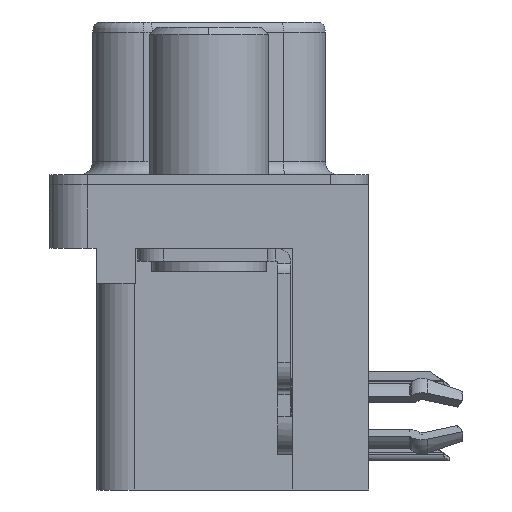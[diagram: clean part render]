
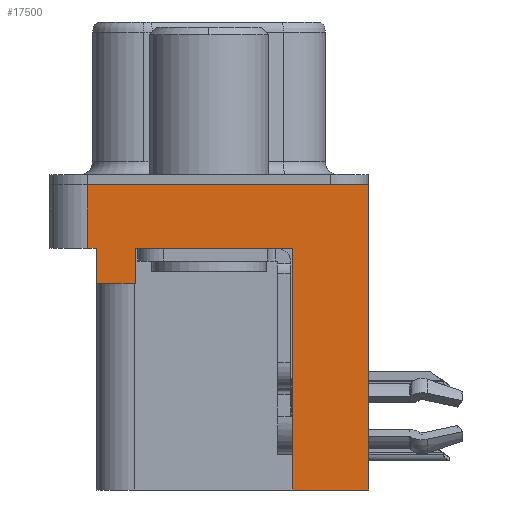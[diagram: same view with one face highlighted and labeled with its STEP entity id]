
A CAD part, left-side view. The second image highlights one B-rep face of the part: STEP entity #17500.
In plain terms, the highlighted planar face has unit normal (-1, 0, 0).
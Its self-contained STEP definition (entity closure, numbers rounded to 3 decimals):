
#219 = AXIS2_PLACEMENT_3D ( 'NONE', #14425, #825, #19557 ) ;
#487 = CARTESIAN_POINT ( 'NONE',  ( -3., 4.775, 0. ) ) ;
#608 = CARTESIAN_POINT ( 'NONE',  ( -3., 4.425, -2.5 ) ) ;
#825 = DIRECTION ( 'NONE',  ( -1., 0., 0. ) ) ;
#910 = VECTOR ( 'NONE', #11393, 1000. ) ;
#1027 = LINE ( 'NONE', #5303, #11777 ) ;
#1289 = ORIENTED_EDGE ( 'NONE', *, *, #22058, .T. ) ;
#1458 = DIRECTION ( 'NONE',  ( 0., -1., 0. ) ) ;
#1572 = EDGE_LOOP ( 'NONE', ( #5381, #14728, #16330, #17282, #4037, #6129, #1289, #3602, #12675, #18749 ) ) ;
#2062 = DIRECTION ( 'NONE',  ( 0., 0., 1. ) ) ;
#2602 = VERTEX_POINT ( 'NONE', #22651 ) ;
#3520 = VERTEX_POINT ( 'NONE', #20927 ) ;
#3602 = ORIENTED_EDGE ( 'NONE', *, *, #14326, .F. ) ;
#4037 = ORIENTED_EDGE ( 'NONE', *, *, #7363, .F. ) ;
#4513 = EDGE_CURVE ( 'NONE', #12724, #22616, #8514, .T. ) ;
#4618 = CARTESIAN_POINT ( 'NONE',  ( -3., -3.295, -12. ) ) ;
#5106 = VECTOR ( 'NONE', #17898, 1000. ) ;
#5303 = CARTESIAN_POINT ( 'NONE',  ( -3., -6.275, -2.5 ) ) ;
#5381 = ORIENTED_EDGE ( 'NONE', *, *, #9587, .F. ) ;
#5887 = CARTESIAN_POINT ( 'NONE',  ( -3., 2.895, -3.9 ) ) ;
#6129 = ORIENTED_EDGE ( 'NONE', *, *, #20632, .T. ) ;
#6624 = DIRECTION ( 'NONE',  ( 0., 1., 0. ) ) ;
#6923 = DIRECTION ( 'NONE',  ( 0., -1., 0. ) ) ;
#6951 = DIRECTION ( 'NONE',  ( 0., 0., 1. ) ) ;
#7041 = CARTESIAN_POINT ( 'NONE',  ( -3., 4.425, -3.9 ) ) ;
#7279 = CARTESIAN_POINT ( 'NONE',  ( -3., -3.295, -12. ) ) ;
#7363 = EDGE_CURVE ( 'NONE', #14541, #21004, #24145, .T. ) ;
#8294 = DIRECTION ( 'NONE',  ( 0., 1., 0. ) ) ;
#8514 = LINE ( 'NONE', #4618, #14204 ) ;
#9392 = EDGE_CURVE ( 'NONE', #18677, #16371, #24678, .T. ) ;
#9587 = EDGE_CURVE ( 'NONE', #16371, #19095, #24375, .T. ) ;
#9686 = CARTESIAN_POINT ( 'NONE',  ( -3., -6.275, 0. ) ) ;
#9701 = FACE_OUTER_BOUND ( 'NONE', #1572, .T. ) ;
#9835 = PLANE ( 'NONE',  #219 ) ;
#9888 = CARTESIAN_POINT ( 'NONE',  ( -3., 4.775, -2.5 ) ) ;
#10728 = VECTOR ( 'NONE', #6923, 1000. ) ;
#11393 = DIRECTION ( 'NONE',  ( 0., 0., 1. ) ) ;
#11777 = VECTOR ( 'NONE', #6951, 1000. ) ;
#11969 = CARTESIAN_POINT ( 'NONE',  ( -3., 4.775, -2.5 ) ) ;
#12283 = CARTESIAN_POINT ( 'NONE',  ( -3., 4.425, -3.9 ) ) ;
#12320 = EDGE_CURVE ( 'NONE', #21004, #18880, #13781, .T. ) ;
#12675 = ORIENTED_EDGE ( 'NONE', *, *, #4513, .F. ) ;
#12724 = VERTEX_POINT ( 'NONE', #24806 ) ;
#12850 = CARTESIAN_POINT ( 'NONE',  ( -3., 2.895, -3.9 ) ) ;
#12912 = CARTESIAN_POINT ( 'NONE',  ( -3., -6.275, 0. ) ) ;
#13331 = EDGE_CURVE ( 'NONE', #18677, #18880, #19086, .T. ) ;
#13781 = LINE ( 'NONE', #22675, #910 ) ;
#13825 = EDGE_CURVE ( 'NONE', #12724, #19095, #1027, .T. ) ;
#14089 = DIRECTION ( 'NONE',  ( 0., 0., 1. ) ) ;
#14204 = VECTOR ( 'NONE', #8294, 1000. ) ;
#14326 = EDGE_CURVE ( 'NONE', #22616, #2602, #20299, .T. ) ;
#14425 = CARTESIAN_POINT ( 'NONE',  ( -3., -6.275, -2.5 ) ) ;
#14541 = VERTEX_POINT ( 'NONE', #5887 ) ;
#14728 = ORIENTED_EDGE ( 'NONE', *, *, #9392, .F. ) ;
#14796 = VECTOR ( 'NONE', #1458, 1000. ) ;
#14820 = DIRECTION ( 'NONE',  ( 0., 0., 1. ) ) ;
#16330 = ORIENTED_EDGE ( 'NONE', *, *, #13331, .T. ) ;
#16371 = VERTEX_POINT ( 'NONE', #487 ) ;
#16472 = CARTESIAN_POINT ( 'NONE',  ( -3., -6.275, -2.5 ) ) ;
#17282 = ORIENTED_EDGE ( 'NONE', *, *, #12320, .F. ) ;
#17312 = CARTESIAN_POINT ( 'NONE',  ( -3., -3.295, -12. ) ) ;
#17500 = ADVANCED_FACE ( 'NONE', ( #9701 ), #9835, .T. ) ;
#17898 = DIRECTION ( 'NONE',  ( 0., -1., 0. ) ) ;
#18480 = VECTOR ( 'NONE', #6624, 1000. ) ;
#18677 = VERTEX_POINT ( 'NONE', #11969 ) ;
#18749 = ORIENTED_EDGE ( 'NONE', *, *, #13825, .T. ) ;
#18880 = VERTEX_POINT ( 'NONE', #608 ) ;
#19086 = LINE ( 'NONE', #16472, #10728 ) ;
#19095 = VERTEX_POINT ( 'NONE', #9686 ) ;
#19134 = VECTOR ( 'NONE', #2062, 1000. ) ;
#19557 = DIRECTION ( 'NONE',  ( 0., 0., 1. ) ) ;
#19733 = LINE ( 'NONE', #23632, #5106 ) ;
#19889 = VECTOR ( 'NONE', #14089, 1000. ) ;
#20299 = LINE ( 'NONE', #7279, #21797 ) ;
#20632 = EDGE_CURVE ( 'NONE', #14541, #3520, #24256, .T. ) ;
#20927 = CARTESIAN_POINT ( 'NONE',  ( -3., 2.895, -2.5 ) ) ;
#21004 = VERTEX_POINT ( 'NONE', #7041 ) ;
#21797 = VECTOR ( 'NONE', #14820, 1000. ) ;
#22058 = EDGE_CURVE ( 'NONE', #3520, #2602, #19733, .T. ) ;
#22616 = VERTEX_POINT ( 'NONE', #17312 ) ;
#22651 = CARTESIAN_POINT ( 'NONE',  ( -3., -3.295, -2.5 ) ) ;
#22675 = CARTESIAN_POINT ( 'NONE',  ( -3., 4.425, -3.9 ) ) ;
#23632 = CARTESIAN_POINT ( 'NONE',  ( -3., -6.275, -2.5 ) ) ;
#24145 = LINE ( 'NONE', #12283, #18480 ) ;
#24256 = LINE ( 'NONE', #12850, #19134 ) ;
#24375 = LINE ( 'NONE', #12912, #14796 ) ;
#24678 = LINE ( 'NONE', #9888, #19889 ) ;
#24806 = CARTESIAN_POINT ( 'NONE',  ( -3., -6.275, -12. ) ) ;
